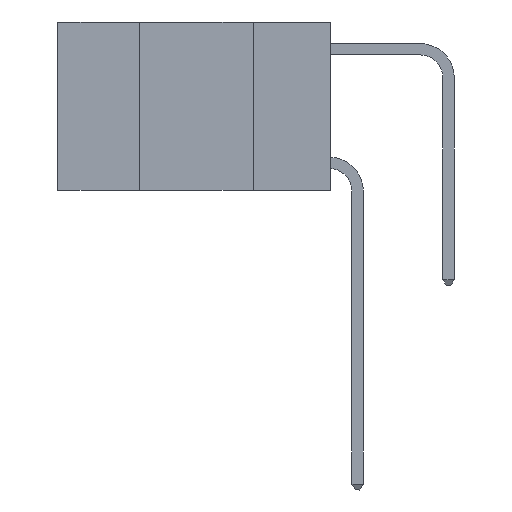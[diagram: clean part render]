
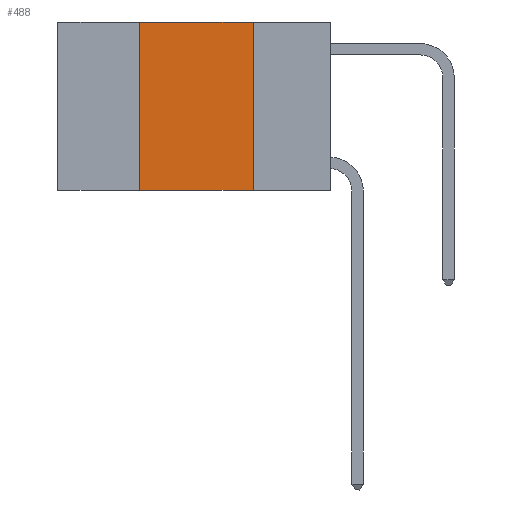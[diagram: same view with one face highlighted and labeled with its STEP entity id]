
A CAD part, left-side view. The second image highlights one B-rep face of the part: STEP entity #488.
In plain terms, the highlighted planar face has unit normal (-1, 0, 0).
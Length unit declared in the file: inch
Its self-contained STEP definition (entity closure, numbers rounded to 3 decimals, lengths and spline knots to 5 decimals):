
#26 = CARTESIAN_POINT ( 'NONE',  ( 0., 0.6, 0. ) ) ;
#401 = DIRECTION ( 'NONE',  ( 0., 0., -1. ) ) ;
#488 = ADVANCED_FACE ( 'NONE', ( #3077 ), #6178, .F. ) ;
#752 = EDGE_CURVE ( 'NONE', #5891, #4225, #11118, .T. ) ;
#1097 = EDGE_CURVE ( 'NONE', #9647, #8037, #7348, .T. ) ;
#1337 = LINE ( 'NONE', #5521, #5106 ) ;
#2088 = CARTESIAN_POINT ( 'NONE',  ( 0., 0.6, 0. ) ) ;
#3077 = FACE_OUTER_BOUND ( 'NONE', #9763, .T. ) ;
#3743 = LINE ( 'NONE', #9880, #6042 ) ;
#4225 = VERTEX_POINT ( 'NONE', #10491 ) ;
#4376 = CARTESIAN_POINT ( 'NONE',  ( 0., 0.42, -0.37 ) ) ;
#4811 = DIRECTION ( 'NONE',  ( 0., 0., 1. ) ) ;
#4848 = ORIENTED_EDGE ( 'NONE', *, *, #1097, .T. ) ;
#5106 = VECTOR ( 'NONE', #401, 39.37008 ) ;
#5374 = AXIS2_PLACEMENT_3D ( 'NONE', #26, #10325, #8206 ) ;
#5521 = CARTESIAN_POINT ( 'NONE',  ( 0., 0.17, 0. ) ) ;
#5891 = VERTEX_POINT ( 'NONE', #10775 ) ;
#6042 = VECTOR ( 'NONE', #4811, 39.37008 ) ;
#6044 = ORIENTED_EDGE ( 'NONE', *, *, #11286, .F. ) ;
#6178 = PLANE ( 'NONE',  #5374 ) ;
#6517 = VECTOR ( 'NONE', #10099, 39.37008 ) ;
#6699 = DIRECTION ( 'NONE',  ( 0., -1., 0. ) ) ;
#7348 = LINE ( 'NONE', #7723, #9323 ) ;
#7505 = ORIENTED_EDGE ( 'NONE', *, *, #752, .F. ) ;
#7575 = CARTESIAN_POINT ( 'NONE',  ( 0., 0.17, -0.37 ) ) ;
#7723 = CARTESIAN_POINT ( 'NONE',  ( 0., 0.6, -0.37 ) ) ;
#8037 = VERTEX_POINT ( 'NONE', #7575 ) ;
#8206 = DIRECTION ( 'NONE',  ( 0., 0., -1. ) ) ;
#9323 = VECTOR ( 'NONE', #6699, 39.37008 ) ;
#9511 = ORIENTED_EDGE ( 'NONE', *, *, #12924, .F. ) ;
#9647 = VERTEX_POINT ( 'NONE', #4376 ) ;
#9763 = EDGE_LOOP ( 'NONE', ( #6044, #7505, #9511, #4848 ) ) ;
#9880 = CARTESIAN_POINT ( 'NONE',  ( 0., 0.42, 0. ) ) ;
#10099 = DIRECTION ( 'NONE',  ( 0., -1., 0. ) ) ;
#10325 = DIRECTION ( 'NONE',  ( 1., 0., 0. ) ) ;
#10491 = CARTESIAN_POINT ( 'NONE',  ( 0., 0.17, 0. ) ) ;
#10775 = CARTESIAN_POINT ( 'NONE',  ( 0., 0.42, 0. ) ) ;
#11118 = LINE ( 'NONE', #2088, #6517 ) ;
#11286 = EDGE_CURVE ( 'NONE', #4225, #8037, #1337, .T. ) ;
#12924 = EDGE_CURVE ( 'NONE', #9647, #5891, #3743, .T. ) ;
